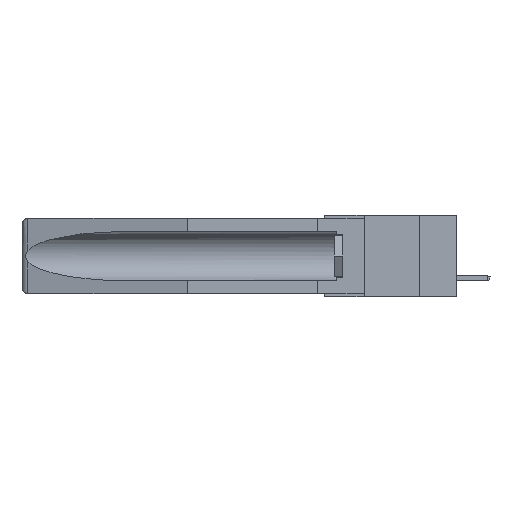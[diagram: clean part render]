
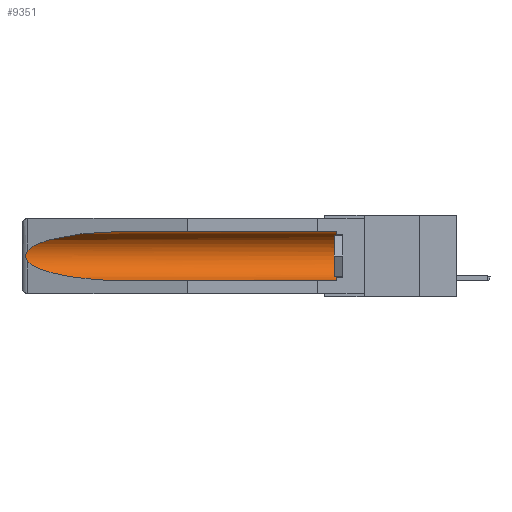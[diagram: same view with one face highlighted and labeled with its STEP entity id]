
A CAD part, left-side view. The second image highlights one B-rep face of the part: STEP entity #9351.
In plain terms, the highlighted cylindrical face has radius 2.857 mm (diameter 5.715 mm), a partial arc.
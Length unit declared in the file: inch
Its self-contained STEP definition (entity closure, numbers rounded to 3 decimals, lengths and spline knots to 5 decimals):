
#173 = CARTESIAN_POINT ( 'NONE',  ( 0.155, -0.30754, -0.1715 ) ) ;
#549 = VERTEX_POINT ( 'NONE', #24330 ) ;
#583 = CARTESIAN_POINT ( 'NONE',  ( 0.155, 1.07973, -0.059 ) ) ;
#866 = CARTESIAN_POINT ( 'NONE',  ( 0.2673, 1.53269, -0.17917 ) ) ;
#2687 = AXIS2_PLACEMENT_3D ( 'NONE', #4315, #4576, #12692 ) ;
#2708 = CARTESIAN_POINT ( 'NONE',  ( 0.25451, 1.48313, -0.09465 ) ) ;
#3103 = VECTOR ( 'NONE', #20217, 39.37008 ) ;
#3337 = CARTESIAN_POINT ( 'NONE',  ( 0.155, 1.07973, -0.284 ) ) ;
#4032 = CARTESIAN_POINT ( 'NONE',  ( 0.26537, 1.52718, -0.19328 ) ) ;
#4315 = CARTESIAN_POINT ( 'NONE',  ( 0.155, 0.126, -0.1715 ) ) ;
#4576 = DIRECTION ( 'NONE',  ( 0., -1., 0. ) ) ;
#6263 = DIRECTION ( 'NONE',  ( 0., 1., 0. ) ) ;
#6382 = ORIENTED_EDGE ( 'NONE', *, *, #20278, .F. ) ;
#6412 = EDGE_CURVE ( 'NONE', #549, #21209, #9121, .T. ) ;
#6603 = ORIENTED_EDGE ( 'NONE', *, *, #21598, .T. ) ;
#6840 = EDGE_CURVE ( 'NONE', #20226, #18023, #17014, .T. ) ;
#7098 = CARTESIAN_POINT ( 'NONE',  ( 0.26597, 1.52961, -0.15275 ) ) ;
#7962 = EDGE_CURVE ( 'NONE', #18023, #549, #17609, .T. ) ;
#8009 = CARTESIAN_POINT ( 'NONE',  ( 0.155, 0.126, -0.284 ) ) ;
#8296 = CYLINDRICAL_SURFACE ( 'NONE', #17935, 0.1125 ) ;
#8443 = CARTESIAN_POINT ( 'NONE',  ( 0.155, 1.07973, -0.284 ) ) ;
#9071 = CARTESIAN_POINT ( 'NONE',  ( 0.155, 0.126, -0.059 ) ) ;
#9121 =( BOUNDED_CURVE ( )  B_SPLINE_CURVE ( 3, ( #583, #23493, #2708, #25612 ),
 .UNSPECIFIED., .F., .F. ) 
 B_SPLINE_CURVE_WITH_KNOTS ( ( 4, 4 ),
 ( 4.71239, 6.08839 ),
 .UNSPECIFIED. ) 
 CURVE ( )  GEOMETRIC_REPRESENTATION_ITEM ( )  RATIONAL_B_SPLINE_CURVE ( ( 1., 0.848, 0.848, 1. ) ) 
 REPRESENTATION_ITEM ( '' )  );
#9175 = CARTESIAN_POINT ( 'NONE',  ( 0.2675, 1.53308, -0.16763 ) ) ;
#9351 = ADVANCED_FACE ( 'NONE', ( #22318 ), #8296, .F. ) ;
#10649 = DIRECTION ( 'NONE',  ( 0., 0., 1. ) ) ;
#11200 = ORIENTED_EDGE ( 'NONE', *, *, #7962, .T. ) ;
#11290 = LINE ( 'NONE', #16026, #3103 ) ;
#11539 = CARTESIAN_POINT ( 'NONE',  ( 0.26597, 1.5296, -0.19026 ) ) ;
#12692 = DIRECTION ( 'NONE',  ( 0., 0., 1. ) ) ;
#13011 = ORIENTED_EDGE ( 'NONE', *, *, #6840, .T. ) ;
#13454 = CARTESIAN_POINT ( 'NONE',  ( 0.26655, 1.53094, -0.18657 ) ) ;
#14380 = DIRECTION ( 'NONE',  ( 0., 1., 0. ) ) ;
#15557 = CARTESIAN_POINT ( 'NONE',  ( 0.26537, 1.52718, -0.19328 ) ) ;
#16026 = CARTESIAN_POINT ( 'NONE',  ( 0.155, -0.30754, -0.284 ) ) ;
#16165 = CARTESIAN_POINT ( 'NONE',  ( 0.26537, 1.52718, -0.19328 ) ) ;
#16632 = CARTESIAN_POINT ( 'NONE',  ( 0.155, -0.30754, -0.059 ) ) ;
#17014 = CIRCLE ( 'NONE', #2687, 0.1125 ) ;
#17094 = CARTESIAN_POINT ( 'NONE',  ( 0.21114, 1.30732, -0.284 ) ) ;
#17384 = EDGE_LOOP ( 'NONE', ( #25558, #22033, #6603, #6382, #13011, #11200 ) ) ;
#17434 = EDGE_CURVE ( 'NONE', #21209, #26213, #24877, .T. ) ;
#17495 = CARTESIAN_POINT ( 'NONE',  ( 0.26537, 1.52718, -0.14972 ) ) ;
#17609 = LINE ( 'NONE', #16632, #22161 ) ;
#17935 = AXIS2_PLACEMENT_3D ( 'NONE', #173, #14380, #10649 ) ;
#18005 =( BOUNDED_CURVE ( )  B_SPLINE_CURVE ( 3, ( #4032, #21195, #17094, #8443 ),
 .UNSPECIFIED., .F., .F. ) 
 B_SPLINE_CURVE_WITH_KNOTS ( ( 4, 4 ),
 ( 0.1948, 1.5708 ),
 .UNSPECIFIED. ) 
 CURVE ( )  GEOMETRIC_REPRESENTATION_ITEM ( )  RATIONAL_B_SPLINE_CURVE ( ( 1., 0.848, 0.848, 1. ) ) 
 REPRESENTATION_ITEM ( '' )  );
#18023 = VERTEX_POINT ( 'NONE', #9071 ) ;
#19511 = CARTESIAN_POINT ( 'NONE',  ( 0.2673, 1.5327, -0.16383 ) ) ;
#20217 = DIRECTION ( 'NONE',  ( 0., 1., 0. ) ) ;
#20226 = VERTEX_POINT ( 'NONE', #8009 ) ;
#20278 = EDGE_CURVE ( 'NONE', #20226, #25235, #11290, .T. ) ;
#21195 = CARTESIAN_POINT ( 'NONE',  ( 0.25451, 1.48313, -0.24835 ) ) ;
#21209 = VERTEX_POINT ( 'NONE', #25725 ) ;
#21598 = EDGE_CURVE ( 'NONE', #26213, #25235, #18005, .T. ) ;
#21681 = CARTESIAN_POINT ( 'NONE',  ( 0.26654, 1.53092, -0.15636 ) ) ;
#22033 = ORIENTED_EDGE ( 'NONE', *, *, #17434, .T. ) ;
#22161 = VECTOR ( 'NONE', #6263, 39.37008 ) ;
#22318 = FACE_OUTER_BOUND ( 'NONE', #17384, .T. ) ;
#23493 = CARTESIAN_POINT ( 'NONE',  ( 0.21114, 1.30732, -0.059 ) ) ;
#23969 = CARTESIAN_POINT ( 'NONE',  ( 0.2675, 1.53308, -0.17534 ) ) ;
#24330 = CARTESIAN_POINT ( 'NONE',  ( 0.155, 1.07973, -0.059 ) ) ;
#24877 = B_SPLINE_CURVE_WITH_KNOTS ( 'NONE', 3,
 ( #17495, #7098, #21681, #19511, #9175, #23969, #866, #13454, #11539, #15557 ),
 .UNSPECIFIED., .F., .F.,
 ( 4, 2, 2, 2, 4 ),
 ( 0., 0.00029, 0.00058, 0.00087, 0.00117 ),
 .UNSPECIFIED. ) ;
#25235 = VERTEX_POINT ( 'NONE', #3337 ) ;
#25558 = ORIENTED_EDGE ( 'NONE', *, *, #6412, .T. ) ;
#25612 = CARTESIAN_POINT ( 'NONE',  ( 0.26537, 1.52718, -0.14972 ) ) ;
#25725 = CARTESIAN_POINT ( 'NONE',  ( 0.26537, 1.52718, -0.14972 ) ) ;
#26213 = VERTEX_POINT ( 'NONE', #16165 ) ;
